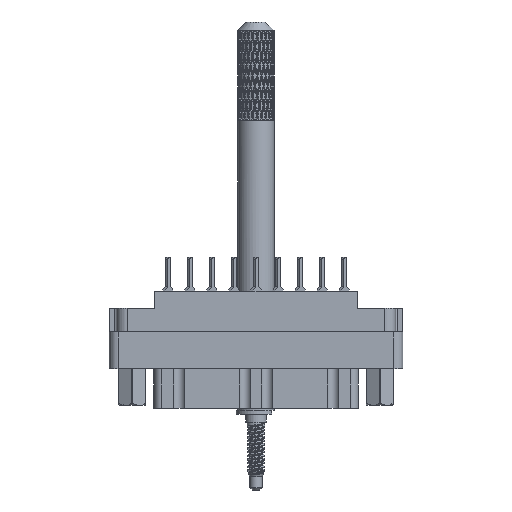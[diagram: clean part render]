
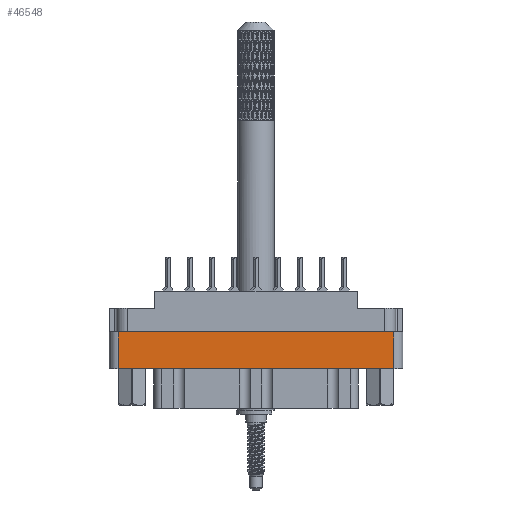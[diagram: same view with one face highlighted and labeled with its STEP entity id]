
A CAD part, front view. The second image highlights one B-rep face of the part: STEP entity #46548.
In plain terms, the highlighted planar face has unit normal (0, -1, 0).
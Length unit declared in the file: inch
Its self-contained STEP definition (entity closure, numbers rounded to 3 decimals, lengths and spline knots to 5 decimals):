
#4250 = ORIENTED_EDGE ( 'NONE', *, *, #94600, .T. ) ;
#7628 = VERTEX_POINT ( 'NONE', #35979 ) ;
#10332 = VECTOR ( 'NONE', #20275, 39.37008 ) ;
#12290 = PLANE ( 'NONE',  #44937 ) ;
#20275 = DIRECTION ( 'NONE',  ( 1., 0., 0. ) ) ;
#21775 = CARTESIAN_POINT ( 'NONE',  ( -0.938, -0.438, -0.798 ) ) ;
#21872 = DIRECTION ( 'NONE',  ( -1., 0., 0. ) ) ;
#23898 = CARTESIAN_POINT ( 'NONE',  ( 0.938, -0.438, -0.277 ) ) ;
#26023 = VECTOR ( 'NONE', #21872, 39.37008 ) ;
#28798 = VECTOR ( 'NONE', #91574, 39.37008 ) ;
#35979 = CARTESIAN_POINT ( 'NONE',  ( 0.938, -0.438, -0.529 ) ) ;
#36954 = EDGE_LOOP ( 'NONE', ( #68820, #97361, #4250, #81824 ) ) ;
#38327 = EDGE_CURVE ( 'NONE', #39510, #109936, #45496, .T. ) ;
#39510 = VERTEX_POINT ( 'NONE', #43734 ) ;
#39789 = CARTESIAN_POINT ( 'NONE',  ( 0.938, -0.438, -0.529 ) ) ;
#42954 = CARTESIAN_POINT ( 'NONE',  ( -0.938, -0.438, -0.529 ) ) ;
#43734 = CARTESIAN_POINT ( 'NONE',  ( -0.938, -0.438, -0.277 ) ) ;
#44210 = VECTOR ( 'NONE', #98185, 39.37008 ) ;
#44937 = AXIS2_PLACEMENT_3D ( 'NONE', #21775, #74466, #107001 ) ;
#44946 = CARTESIAN_POINT ( 'NONE',  ( -1., -0.438, -0.277 ) ) ;
#45496 = LINE ( 'NONE', #44946, #10332 ) ;
#46548 = ADVANCED_FACE ( 'NONE', ( #89070 ), #12290, .T. ) ;
#57353 = CARTESIAN_POINT ( 'NONE',  ( -0.938, -0.438, -0.798 ) ) ;
#62305 = CARTESIAN_POINT ( 'NONE',  ( 0.938, -0.438, -0.798 ) ) ;
#68820 = ORIENTED_EDGE ( 'NONE', *, *, #104518, .F. ) ;
#70044 = EDGE_CURVE ( 'NONE', #7628, #100556, #80744, .T. ) ;
#74466 = DIRECTION ( 'NONE',  ( 0., -1., 0. ) ) ;
#79686 = LINE ( 'NONE', #62305, #44210 ) ;
#80744 = LINE ( 'NONE', #39789, #26023 ) ;
#81824 = ORIENTED_EDGE ( 'NONE', *, *, #38327, .F. ) ;
#83158 = LINE ( 'NONE', #57353, #28798 ) ;
#89070 = FACE_OUTER_BOUND ( 'NONE', #36954, .T. ) ;
#91574 = DIRECTION ( 'NONE',  ( 0., 0., 1. ) ) ;
#94600 = EDGE_CURVE ( 'NONE', #7628, #109936, #79686, .T. ) ;
#97361 = ORIENTED_EDGE ( 'NONE', *, *, #70044, .F. ) ;
#98185 = DIRECTION ( 'NONE',  ( 0., 0., 1. ) ) ;
#100556 = VERTEX_POINT ( 'NONE', #42954 ) ;
#104518 = EDGE_CURVE ( 'NONE', #100556, #39510, #83158, .T. ) ;
#107001 = DIRECTION ( 'NONE',  ( 0., 0., -1. ) ) ;
#109936 = VERTEX_POINT ( 'NONE', #23898 ) ;
